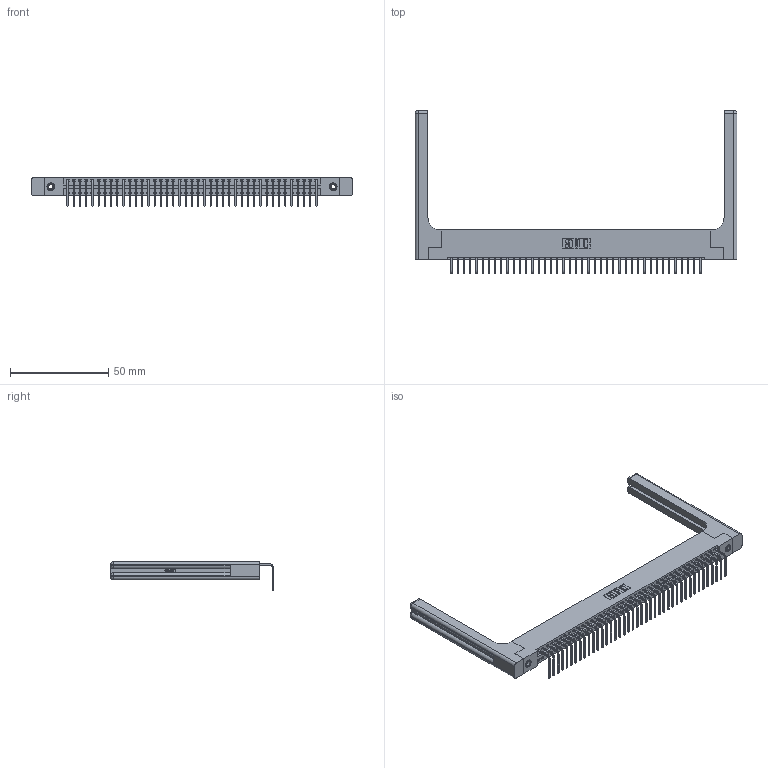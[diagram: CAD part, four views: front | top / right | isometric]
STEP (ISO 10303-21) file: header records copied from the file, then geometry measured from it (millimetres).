
FILE_DESCRIPTION (( 'STEP AP203' ), '1' );
FILE_NAME ('396-041-558-158.STEP', '2019-11-01T07:50:47', ( '' ), ( '' ), 'SwSTEP 2.0', 'SolidWorks 2016', '' );
FILE_SCHEMA (( 'CONFIG_CONTROL_DESIGN' ));
Length unit declared in the file: inch
Products named in the file (5): 396-041-558-158; 346 Part_Flush Mounting Lugs - 0.156 Dia-TH; 345-292-001_558 Tail - 2; 345-250-001_345-250-001-102; 346-220-058_345-220-058
Assembly tree (46 placements, depth 2):
  396-041-558-158
    346 Part_Flush Mounting Lugs - 0.156 Dia-TH
    345-292-001_558 Tail - 2  x41
    345-250-001_345-250-001-102  x2
    346-220-058_345-220-058  x2
Bounding box: 164.24 x 83.12 x 14.73 mm (x, y, z)
Volume: 23369.2 mm3; surface area: 25785.1 mm2
Topology: 46 solids, 46 shells, 2838 faces, 8457 edges, 5562 vertices
Faces by surface type: plane 1946, cylinder 832, bspline 36, cone 12, sphere 8, torus 4
Entity records: 30846 total; most frequent: CARTESIAN_POINT 6268, ORIENTED_EDGE 5040, DIRECTION 4462, EDGE_CURVE 2520, LINE 2132, VECTOR 2132, VERTEX_POINT 1670, AXIS2_PLACEMENT_3D 1165
